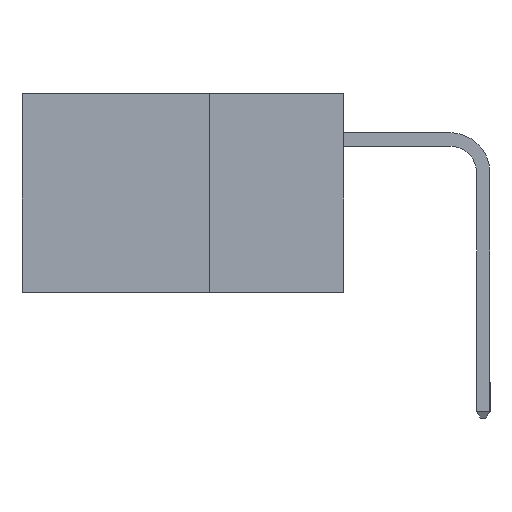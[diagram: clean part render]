
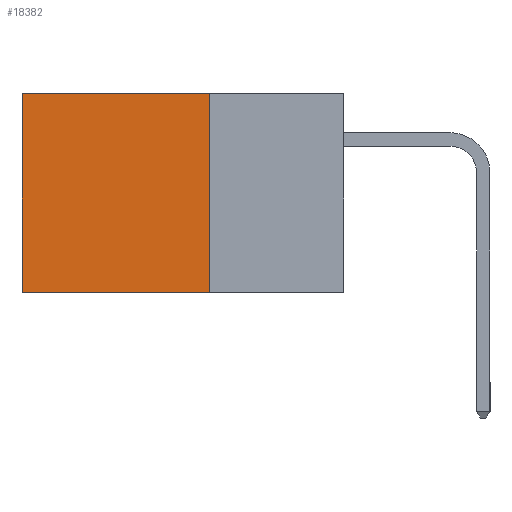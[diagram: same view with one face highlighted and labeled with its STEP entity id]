
A CAD part, left-side view. The second image highlights one B-rep face of the part: STEP entity #18382.
In plain terms, the highlighted planar face has unit normal (-1, 0, 0).
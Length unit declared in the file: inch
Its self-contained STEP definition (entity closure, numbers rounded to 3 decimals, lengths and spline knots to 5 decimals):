
#796 = CARTESIAN_POINT ( 'NONE',  ( 0.298, 0.25, -0.37 ) ) ;
#803 = EDGE_CURVE ( 'NONE', #10755, #1880, #864, .T. ) ;
#864 = LINE ( 'NONE', #1388, #20320 ) ;
#979 = CARTESIAN_POINT ( 'NONE',  ( 0.298, 0.25, 0. ) ) ;
#1190 = PLANE ( 'NONE',  #5696 ) ;
#1388 = CARTESIAN_POINT ( 'NONE',  ( 0.298, 0.25, 0. ) ) ;
#1880 = VERTEX_POINT ( 'NONE', #796 ) ;
#3048 = DIRECTION ( 'NONE',  ( 0., 1., 0. ) ) ;
#3123 = ORIENTED_EDGE ( 'NONE', *, *, #5211, .T. ) ;
#4285 = VECTOR ( 'NONE', #14077, 39.37008 ) ;
#5152 = DIRECTION ( 'NONE',  ( 1., 0., 0. ) ) ;
#5211 = EDGE_CURVE ( 'NONE', #14436, #7150, #14624, .T. ) ;
#5696 = AXIS2_PLACEMENT_3D ( 'NONE', #14837, #5152, #18708 ) ;
#5720 = FACE_OUTER_BOUND ( 'NONE', #16348, .T. ) ;
#6210 = LINE ( 'NONE', #22443, #15286 ) ;
#6352 = VECTOR ( 'NONE', #3048, 39.37008 ) ;
#6630 = EDGE_CURVE ( 'NONE', #10755, #14436, #12106, .T. ) ;
#7150 = VERTEX_POINT ( 'NONE', #22171 ) ;
#7439 = DIRECTION ( 'NONE',  ( 0., 0., -1. ) ) ;
#8504 = ORIENTED_EDGE ( 'NONE', *, *, #803, .F. ) ;
#10755 = VERTEX_POINT ( 'NONE', #20064 ) ;
#12106 = LINE ( 'NONE', #979, #6352 ) ;
#12119 = CARTESIAN_POINT ( 'NONE',  ( 0.298, 0.6, 0. ) ) ;
#14077 = DIRECTION ( 'NONE',  ( 0., 0., -1. ) ) ;
#14436 = VERTEX_POINT ( 'NONE', #20868 ) ;
#14624 = LINE ( 'NONE', #12119, #4285 ) ;
#14837 = CARTESIAN_POINT ( 'NONE',  ( 0.298, 0.25, 0. ) ) ;
#15286 = VECTOR ( 'NONE', #24376, 39.37008 ) ;
#15976 = ORIENTED_EDGE ( 'NONE', *, *, #6630, .T. ) ;
#16348 = EDGE_LOOP ( 'NONE', ( #3123, #23313, #8504, #15976 ) ) ;
#18382 = ADVANCED_FACE ( 'NONE', ( #5720 ), #1190, .F. ) ;
#18708 = DIRECTION ( 'NONE',  ( 0., 0., -1. ) ) ;
#20064 = CARTESIAN_POINT ( 'NONE',  ( 0.298, 0.25, 0. ) ) ;
#20320 = VECTOR ( 'NONE', #7439, 39.37008 ) ;
#20481 = EDGE_CURVE ( 'NONE', #1880, #7150, #6210, .T. ) ;
#20868 = CARTESIAN_POINT ( 'NONE',  ( 0.298, 0.6, 0. ) ) ;
#22171 = CARTESIAN_POINT ( 'NONE',  ( 0.298, 0.6, -0.37 ) ) ;
#22443 = CARTESIAN_POINT ( 'NONE',  ( 0.298, 0.25, -0.37 ) ) ;
#23313 = ORIENTED_EDGE ( 'NONE', *, *, #20481, .F. ) ;
#24376 = DIRECTION ( 'NONE',  ( 0., 1., 0. ) ) ;
